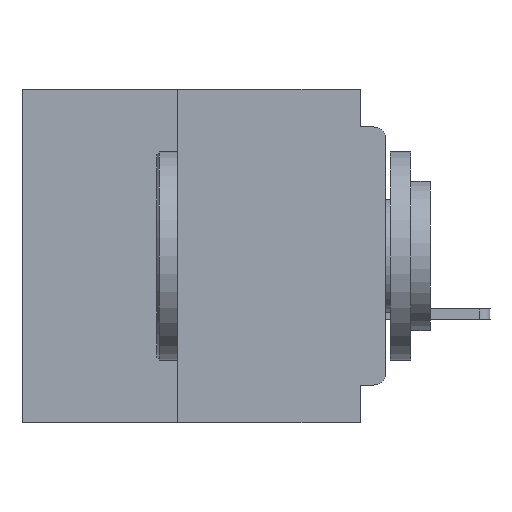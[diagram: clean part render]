
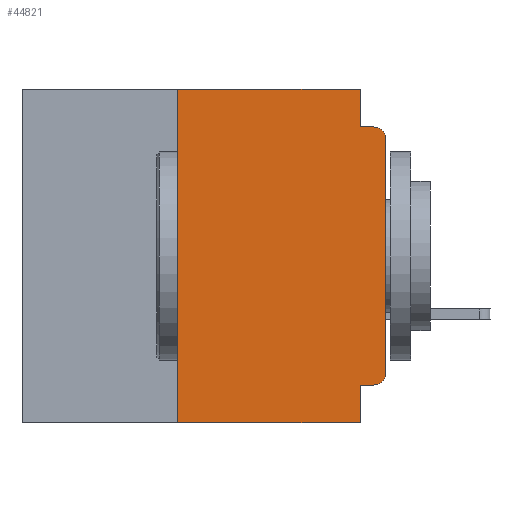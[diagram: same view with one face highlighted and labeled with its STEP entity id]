
A CAD part, left-side view. The second image highlights one B-rep face of the part: STEP entity #44821.
In plain terms, the highlighted planar face has unit normal (-1, 0, 0).
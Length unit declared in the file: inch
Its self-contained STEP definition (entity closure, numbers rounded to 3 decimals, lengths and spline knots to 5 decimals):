
#43 = VERTEX_POINT ( 'NONE', #25123 ) ;
#724 = EDGE_CURVE ( 'NONE', #55753, #43, #10678, .T. ) ;
#1917 = CARTESIAN_POINT ( 'NONE',  ( 0., 0.25, -0.4 ) ) ;
#2105 = DIRECTION ( 'NONE',  ( 0., 0., 1. ) ) ;
#2165 = CARTESIAN_POINT ( 'NONE',  ( 0., 0.437, 0. ) ) ;
#3124 = VECTOR ( 'NONE', #32124, 39.37008 ) ;
#3940 = CARTESIAN_POINT ( 'NONE',  ( 0., 0., -0.06 ) ) ;
#4516 = VECTOR ( 'NONE', #41770, 39.37008 ) ;
#5548 = LINE ( 'NONE', #56813, #14825 ) ;
#5729 = VECTOR ( 'NONE', #2105, 39.37008 ) ;
#5979 = LINE ( 'NONE', #9289, #3124 ) ;
#7306 = EDGE_CURVE ( 'NONE', #55753, #55486, #17844, .T. ) ;
#8628 = EDGE_CURVE ( 'NONE', #45219, #8813, #5548, .T. ) ;
#8717 = ORIENTED_EDGE ( 'NONE', *, *, #54892, .T. ) ;
#8813 = VERTEX_POINT ( 'NONE', #3940 ) ;
#9289 = CARTESIAN_POINT ( 'NONE',  ( 0., 0.031, 0. ) ) ;
#10678 = LINE ( 'NONE', #30500, #34779 ) ;
#10765 = CARTESIAN_POINT ( 'NONE',  ( 0., 0.437, 0. ) ) ;
#10893 = ORIENTED_EDGE ( 'NONE', *, *, #28642, .F. ) ;
#13739 = CARTESIAN_POINT ( 'NONE',  ( 0., 0.015, -0.045 ) ) ;
#13893 = CARTESIAN_POINT ( 'NONE',  ( 0., 0.25, -0.4 ) ) ;
#14825 = VECTOR ( 'NONE', #34135, 39.37008 ) ;
#16498 = CARTESIAN_POINT ( 'NONE',  ( 0., 0.25, 0. ) ) ;
#16768 = ORIENTED_EDGE ( 'NONE', *, *, #51499, .F. ) ;
#16776 = EDGE_CURVE ( 'NONE', #55486, #18927, #54690, .T. ) ;
#17313 = DIRECTION ( 'NONE',  ( -1., 0., 0. ) ) ;
#17844 = LINE ( 'NONE', #1917, #5729 ) ;
#18012 = ORIENTED_EDGE ( 'NONE', *, *, #8628, .T. ) ;
#18047 = DIRECTION ( 'NONE',  ( 0., 1., 0. ) ) ;
#18927 = VERTEX_POINT ( 'NONE', #26947 ) ;
#19006 = CARTESIAN_POINT ( 'NONE',  ( 0., 0., -0.045 ) ) ;
#19857 = ORIENTED_EDGE ( 'NONE', *, *, #724, .T. ) ;
#20491 = ORIENTED_EDGE ( 'NONE', *, *, #26190, .F. ) ;
#21305 = DIRECTION ( 'NONE',  ( 0., 0., -1. ) ) ;
#21900 = CARTESIAN_POINT ( 'NONE',  ( 0., 0.015, -0.06 ) ) ;
#22964 = ORIENTED_EDGE ( 'NONE', *, *, #45281, .F. ) ;
#25123 = CARTESIAN_POINT ( 'NONE',  ( 0., 0.031, -0.4 ) ) ;
#25676 = VERTEX_POINT ( 'NONE', #13739 ) ;
#26190 = EDGE_CURVE ( 'NONE', #18927, #54881, #5979, .T. ) ;
#26457 = DIRECTION ( 'NONE',  ( 0., 0., -1. ) ) ;
#26947 = CARTESIAN_POINT ( 'NONE',  ( 0., 0.031, 0. ) ) ;
#27508 = LINE ( 'NONE', #45216, #38130 ) ;
#28642 = EDGE_CURVE ( 'NONE', #56825, #43, #48922, .T. ) ;
#29009 = DIRECTION ( 'NONE',  ( 0., 0., -1. ) ) ;
#30037 = CARTESIAN_POINT ( 'NONE',  ( 0., 0.031, -0.4 ) ) ;
#30050 = DIRECTION ( 'NONE',  ( 0., -1., 0. ) ) ;
#30500 = CARTESIAN_POINT ( 'NONE',  ( 0., 0.437, -0.4 ) ) ;
#31125 = CARTESIAN_POINT ( 'NONE',  ( 0., 0., -0.34 ) ) ;
#32124 = DIRECTION ( 'NONE',  ( 0., 0., -1. ) ) ;
#33939 = DIRECTION ( 'NONE',  ( 0., -1., 0. ) ) ;
#34135 = DIRECTION ( 'NONE',  ( 0., 0., 1. ) ) ;
#34779 = VECTOR ( 'NONE', #30050, 39.37008 ) ;
#35168 = CARTESIAN_POINT ( 'NONE',  ( 0., 0.031, -0.045 ) ) ;
#35745 = EDGE_LOOP ( 'NONE', ( #18012, #8717, #16768, #20491, #37222, #36080, #19857, #10893, #22964, #37182 ) ) ;
#36080 = ORIENTED_EDGE ( 'NONE', *, *, #7306, .F. ) ;
#36162 = EDGE_CURVE ( 'NONE', #46487, #45219, #52008, .T. ) ;
#36792 = VECTOR ( 'NONE', #21305, 39.37008 ) ;
#37036 = CARTESIAN_POINT ( 'NONE',  ( 0., 0.031, -0.355 ) ) ;
#37182 = ORIENTED_EDGE ( 'NONE', *, *, #36162, .T. ) ;
#37222 = ORIENTED_EDGE ( 'NONE', *, *, #16776, .F. ) ;
#38130 = VECTOR ( 'NONE', #18047, 39.37008 ) ;
#41770 = DIRECTION ( 'NONE',  ( 0., -1., 0. ) ) ;
#42464 = FACE_OUTER_BOUND ( 'NONE', #35745, .T. ) ;
#44490 = CARTESIAN_POINT ( 'NONE',  ( 0., 0.015, -0.34 ) ) ;
#44790 = AXIS2_PLACEMENT_3D ( 'NONE', #10765, #56234, #29009 ) ;
#44821 = ADVANCED_FACE ( 'NONE', ( #42464 ), #51673, .F. ) ;
#45216 = CARTESIAN_POINT ( 'NONE',  ( 0., 0., -0.355 ) ) ;
#45219 = VERTEX_POINT ( 'NONE', #31125 ) ;
#45281 = EDGE_CURVE ( 'NONE', #46487, #56825, #27508, .T. ) ;
#46487 = VERTEX_POINT ( 'NONE', #53670 ) ;
#48856 = CIRCLE ( 'NONE', #58879, 0.015 ) ;
#48922 = LINE ( 'NONE', #30037, #36792 ) ;
#49095 = DIRECTION ( 'NONE',  ( 0., 0., -1. ) ) ;
#51499 = EDGE_CURVE ( 'NONE', #54881, #25676, #54309, .T. ) ;
#51673 = PLANE ( 'NONE',  #44790 ) ;
#51853 = VECTOR ( 'NONE', #33939, 39.37008 ) ;
#52008 = CIRCLE ( 'NONE', #57422, 0.015 ) ;
#53670 = CARTESIAN_POINT ( 'NONE',  ( 0., 0.015, -0.355 ) ) ;
#53692 = DIRECTION ( 'NONE',  ( -1., 0., 0. ) ) ;
#54309 = LINE ( 'NONE', #19006, #4516 ) ;
#54690 = LINE ( 'NONE', #2165, #51853 ) ;
#54881 = VERTEX_POINT ( 'NONE', #35168 ) ;
#54892 = EDGE_CURVE ( 'NONE', #8813, #25676, #48856, .T. ) ;
#55486 = VERTEX_POINT ( 'NONE', #16498 ) ;
#55753 = VERTEX_POINT ( 'NONE', #13893 ) ;
#56234 = DIRECTION ( 'NONE',  ( 1., 0., 0. ) ) ;
#56813 = CARTESIAN_POINT ( 'NONE',  ( 0., 0., 0. ) ) ;
#56825 = VERTEX_POINT ( 'NONE', #37036 ) ;
#57422 = AXIS2_PLACEMENT_3D ( 'NONE', #44490, #17313, #49095 ) ;
#58879 = AXIS2_PLACEMENT_3D ( 'NONE', #21900, #53692, #26457 ) ;
